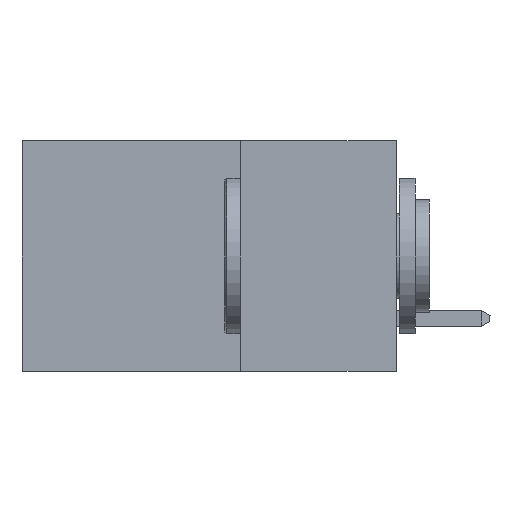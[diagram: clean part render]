
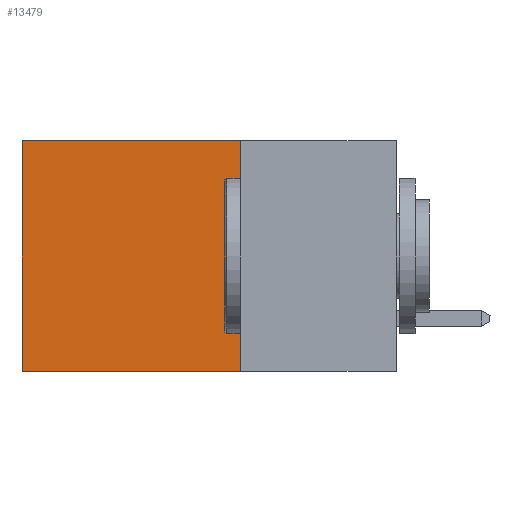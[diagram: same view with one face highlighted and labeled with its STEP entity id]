
A CAD part, left-side view. The second image highlights one B-rep face of the part: STEP entity #13479.
In plain terms, the highlighted planar face has unit normal (-1, 0, 0).
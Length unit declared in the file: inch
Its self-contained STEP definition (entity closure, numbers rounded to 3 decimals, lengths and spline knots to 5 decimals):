
#814 = ORIENTED_EDGE ( 'NONE', *, *, #3065, .F. ) ;
#1052 = CARTESIAN_POINT ( 'NONE',  ( 0.2615, 0.6, -0.37 ) ) ;
#1120 = CARTESIAN_POINT ( 'NONE',  ( 0.2615, 0.25, -0.37 ) ) ;
#1280 = DIRECTION ( 'NONE',  ( 0., 1., 0. ) ) ;
#1294 = DIRECTION ( 'NONE',  ( 0., 0., -1. ) ) ;
#1386 = VERTEX_POINT ( 'NONE', #8055 ) ;
#2570 = DIRECTION ( 'NONE',  ( 0., 0., -1. ) ) ;
#3065 = EDGE_CURVE ( 'NONE', #6937, #1386, #7857, .T. ) ;
#4505 = CARTESIAN_POINT ( 'NONE',  ( 0.2615, 0.25, 0. ) ) ;
#6031 = DIRECTION ( 'NONE',  ( 0., 1., 0. ) ) ;
#6397 = CARTESIAN_POINT ( 'NONE',  ( 0.2615, 0.25, -0.37 ) ) ;
#6446 = ORIENTED_EDGE ( 'NONE', *, *, #12098, .F. ) ;
#6937 = VERTEX_POINT ( 'NONE', #12936 ) ;
#7857 = LINE ( 'NONE', #1120, #15214 ) ;
#8055 = CARTESIAN_POINT ( 'NONE',  ( 0.2615, 0.6, -0.37 ) ) ;
#8166 = ORIENTED_EDGE ( 'NONE', *, *, #14696, .T. ) ;
#8737 = FACE_OUTER_BOUND ( 'NONE', #17346, .T. ) ;
#8956 = CARTESIAN_POINT ( 'NONE',  ( 0.2615, 0.25, -0.37 ) ) ;
#9002 = VECTOR ( 'NONE', #9524, 39.37008 ) ;
#9164 = VECTOR ( 'NONE', #2570, 39.37008 ) ;
#9524 = DIRECTION ( 'NONE',  ( 0., 0., -1. ) ) ;
#10453 = DIRECTION ( 'NONE',  ( 1., 0., 0. ) ) ;
#11711 = VERTEX_POINT ( 'NONE', #17268 ) ;
#11998 = CARTESIAN_POINT ( 'NONE',  ( 0.2615, 0.25, 0. ) ) ;
#12098 = EDGE_CURVE ( 'NONE', #16123, #6937, #16708, .T. ) ;
#12936 = CARTESIAN_POINT ( 'NONE',  ( 0.2615, 0.25, -0.37 ) ) ;
#13205 = EDGE_CURVE ( 'NONE', #16123, #11711, #17983, .T. ) ;
#13479 = ADVANCED_FACE ( 'NONE', ( #8737 ), #17587, .F. ) ;
#14696 = EDGE_CURVE ( 'NONE', #11711, #1386, #16845, .T. ) ;
#14881 = ORIENTED_EDGE ( 'NONE', *, *, #13205, .T. ) ;
#15214 = VECTOR ( 'NONE', #1280, 39.37008 ) ;
#16123 = VERTEX_POINT ( 'NONE', #11998 ) ;
#16222 = AXIS2_PLACEMENT_3D ( 'NONE', #8956, #10453, #1294 ) ;
#16708 = LINE ( 'NONE', #6397, #9002 ) ;
#16845 = LINE ( 'NONE', #1052, #9164 ) ;
#17268 = CARTESIAN_POINT ( 'NONE',  ( 0.2615, 0.6, 0. ) ) ;
#17346 = EDGE_LOOP ( 'NONE', ( #8166, #814, #6446, #14881 ) ) ;
#17553 = VECTOR ( 'NONE', #6031, 39.37008 ) ;
#17587 = PLANE ( 'NONE',  #16222 ) ;
#17983 = LINE ( 'NONE', #4505, #17553 ) ;
